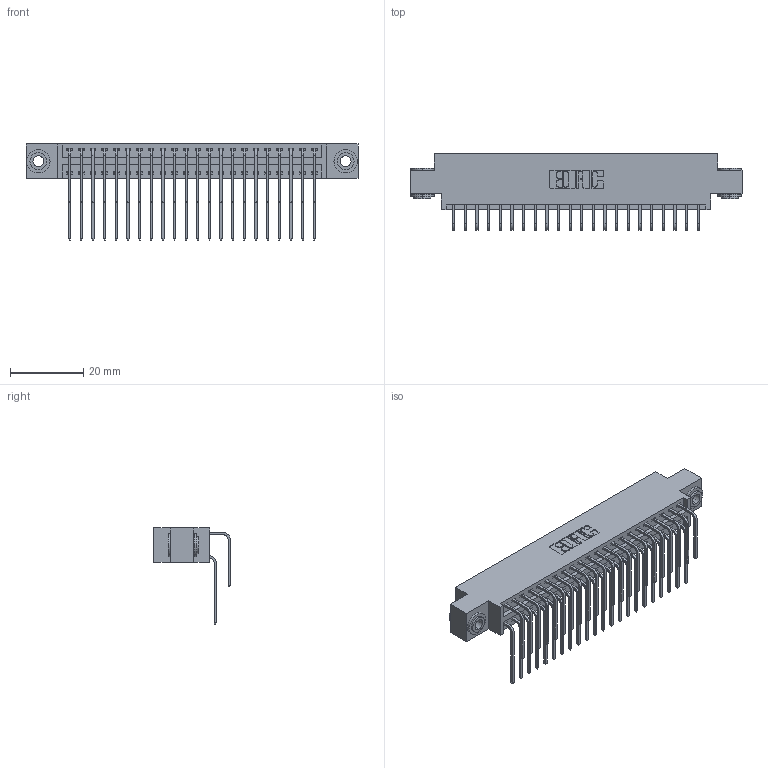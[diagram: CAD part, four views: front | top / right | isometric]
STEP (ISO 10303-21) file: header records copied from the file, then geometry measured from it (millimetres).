
FILE_DESCRIPTION (( 'STEP AP203' ), '1' );
FILE_NAME ('396-044-559-803.STEP', '2018-09-07T05:33:50', ( '' ), ( '' ), 'SwSTEP 2.0', 'SolidWorks 2016', '' );
FILE_SCHEMA (( 'CONFIG_CONTROL_DESIGN' ));
Length unit declared in the file: inch
Products named in the file (5): 345-250-002_345-250-002-102; 396-044-559-803; 346 Part_0.170 Offset - 0.156 Dia-TH; 345-292-001_558 559 Tail - 1; 345-292-001_559 Tail - 2
Assembly tree (47 placements, depth 2):
  396-044-559-803
    346 Part_0.170 Offset - 0.156 Dia-TH
    345-292-001_558 559 Tail - 1  x22
    345-292-001_559 Tail - 2  x22
    345-250-002_345-250-002-102  x2
Bounding box: 90.42 x 20.89 x 26.16 mm (x, y, z)
Volume: 8780.7 mm3; surface area: 13366.8 mm2
Topology: 47 solids, 47 shells, 2540 faces, 7501 edges, 4938 vertices
Faces by surface type: plane 1718, cylinder 814, cone 8
Entity records: 19616 total; most frequent: CARTESIAN_POINT 3290, ORIENTED_EDGE 3166, DIRECTION 2953, EDGE_CURVE 1583, LINE 1299, VECTOR 1299, VERTEX_POINT 1050, AXIS2_PLACEMENT_3D 827
